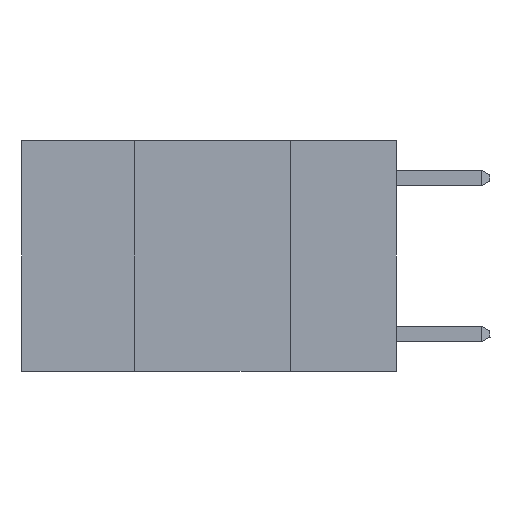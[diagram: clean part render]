
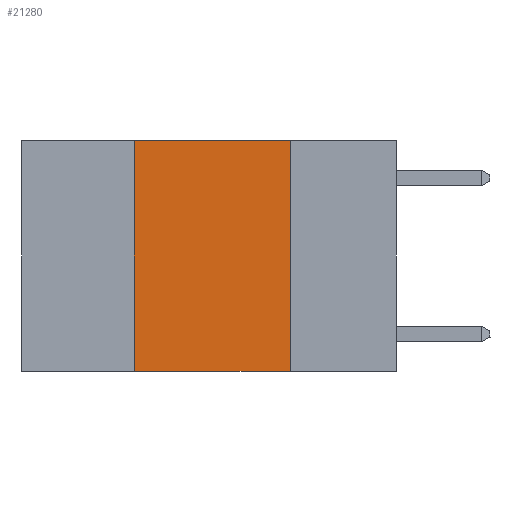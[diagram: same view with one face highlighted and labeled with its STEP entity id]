
A CAD part, left-side view. The second image highlights one B-rep face of the part: STEP entity #21280.
In plain terms, the highlighted planar face has unit normal (-1, 0, 0).
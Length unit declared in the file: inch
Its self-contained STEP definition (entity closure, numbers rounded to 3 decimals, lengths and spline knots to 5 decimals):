
#673 = CARTESIAN_POINT ( 'NONE',  ( 0., 0.42, 0. ) ) ;
#865 = FACE_OUTER_BOUND ( 'NONE', #18092, .T. ) ;
#1187 = CARTESIAN_POINT ( 'NONE',  ( 0., 0.6, -0.37 ) ) ;
#2211 = EDGE_CURVE ( 'NONE', #14963, #2864, #20866, .T. ) ;
#2864 = VERTEX_POINT ( 'NONE', #17017 ) ;
#3638 = DIRECTION ( 'NONE',  ( 1., 0., 0. ) ) ;
#7834 = VECTOR ( 'NONE', #17085, 39.37008 ) ;
#9397 = DIRECTION ( 'NONE',  ( 0., -1., 0. ) ) ;
#9399 = AXIS2_PLACEMENT_3D ( 'NONE', #15645, #3638, #15952 ) ;
#9518 = VERTEX_POINT ( 'NONE', #673 ) ;
#10648 = CARTESIAN_POINT ( 'NONE',  ( 0., 0.42, 0. ) ) ;
#11267 = VECTOR ( 'NONE', #9397, 39.37008 ) ;
#12035 = VECTOR ( 'NONE', #12405, 39.37008 ) ;
#12405 = DIRECTION ( 'NONE',  ( 0., 0., 1. ) ) ;
#12539 = LINE ( 'NONE', #1187, #7834 ) ;
#12866 = ORIENTED_EDGE ( 'NONE', *, *, #2211, .F. ) ;
#14056 = ORIENTED_EDGE ( 'NONE', *, *, #15524, .F. ) ;
#14963 = VERTEX_POINT ( 'NONE', #17949 ) ;
#15412 = CARTESIAN_POINT ( 'NONE',  ( 0., 0.17, 0. ) ) ;
#15484 = DIRECTION ( 'NONE',  ( 0., 0., -1. ) ) ;
#15524 = EDGE_CURVE ( 'NONE', #16378, #9518, #21604, .T. ) ;
#15645 = CARTESIAN_POINT ( 'NONE',  ( 0., 0.6, 0. ) ) ;
#15952 = DIRECTION ( 'NONE',  ( 0., 0., -1. ) ) ;
#16378 = VERTEX_POINT ( 'NONE', #21312 ) ;
#16403 = LINE ( 'NONE', #17996, #11267 ) ;
#16671 = EDGE_CURVE ( 'NONE', #16378, #2864, #12539, .T. ) ;
#17017 = CARTESIAN_POINT ( 'NONE',  ( 0., 0.17, -0.37 ) ) ;
#17085 = DIRECTION ( 'NONE',  ( 0., -1., 0. ) ) ;
#17949 = CARTESIAN_POINT ( 'NONE',  ( 0., 0.17, 0. ) ) ;
#17996 = CARTESIAN_POINT ( 'NONE',  ( 0., 0.6, 0. ) ) ;
#18092 = EDGE_LOOP ( 'NONE', ( #12866, #18339, #14056, #19270 ) ) ;
#18339 = ORIENTED_EDGE ( 'NONE', *, *, #21439, .F. ) ;
#19270 = ORIENTED_EDGE ( 'NONE', *, *, #16671, .T. ) ;
#19337 = VECTOR ( 'NONE', #15484, 39.37008 ) ;
#20866 = LINE ( 'NONE', #15412, #19337 ) ;
#20987 = PLANE ( 'NONE',  #9399 ) ;
#21280 = ADVANCED_FACE ( 'NONE', ( #865 ), #20987, .F. ) ;
#21312 = CARTESIAN_POINT ( 'NONE',  ( 0., 0.42, -0.37 ) ) ;
#21439 = EDGE_CURVE ( 'NONE', #9518, #14963, #16403, .T. ) ;
#21604 = LINE ( 'NONE', #10648, #12035 ) ;
